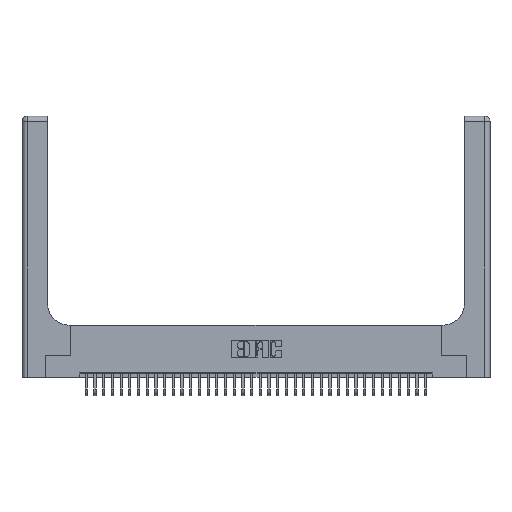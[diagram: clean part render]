
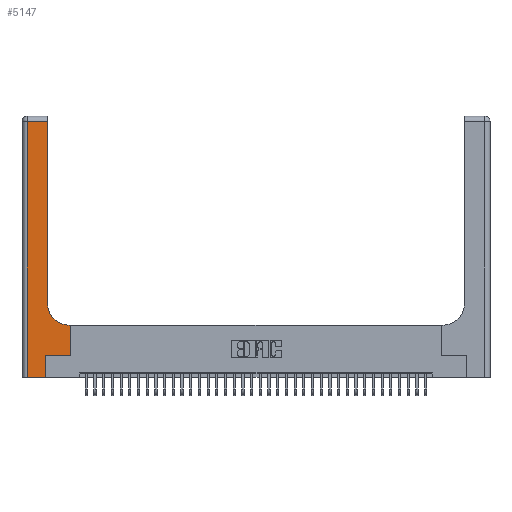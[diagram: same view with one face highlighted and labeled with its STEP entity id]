
A CAD part, top view. The second image highlights one B-rep face of the part: STEP entity #5147.
In plain terms, the highlighted planar face has unit normal (0, 0, 1).
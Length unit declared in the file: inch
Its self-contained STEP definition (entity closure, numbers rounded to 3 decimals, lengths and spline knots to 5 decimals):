
#556 = ORIENTED_EDGE ( 'NONE', *, *, #10678, .T. ) ;
#912 = LINE ( 'NONE', #37851, #16051 ) ;
#923 = VERTEX_POINT ( 'NONE', #15321 ) ;
#1822 = DIRECTION ( 'NONE',  ( 0., 0., -1. ) ) ;
#2585 = EDGE_LOOP ( 'NONE', ( #3251, #27436, #12454, #21646, #556, #5728, #13069, #32507, #8912 ) ) ;
#3251 = ORIENTED_EDGE ( 'NONE', *, *, #26439, .T. ) ;
#5147 = ADVANCED_FACE ( 'NONE', ( #26688 ), #20530, .F. ) ;
#5360 = DIRECTION ( 'NONE',  ( 0., -1., 0. ) ) ;
#5602 = CARTESIAN_POINT ( 'NONE',  ( 0., 3., 0.37 ) ) ;
#5684 = VERTEX_POINT ( 'NONE', #32238 ) ;
#5728 = ORIENTED_EDGE ( 'NONE', *, *, #12887, .T. ) ;
#6260 = AXIS2_PLACEMENT_3D ( 'NONE', #5602, #26417, #8618 ) ;
#6368 = CARTESIAN_POINT ( 'NONE',  ( 0.06, 2.94, 0.37 ) ) ;
#6786 = VECTOR ( 'NONE', #36895, 39.37008 ) ;
#8026 = CARTESIAN_POINT ( 'NONE',  ( 0.5585, 0.6, 0.37 ) ) ;
#8618 = DIRECTION ( 'NONE',  ( -1., 0., 0. ) ) ;
#8731 = LINE ( 'NONE', #11930, #15793 ) ;
#8912 = ORIENTED_EDGE ( 'NONE', *, *, #35461, .T. ) ;
#10533 = CARTESIAN_POINT ( 'NONE',  ( 0.5415, 0.6, 0.37 ) ) ;
#10678 = EDGE_CURVE ( 'NONE', #923, #5684, #22399, .T. ) ;
#11016 = VERTEX_POINT ( 'NONE', #31065 ) ;
#11930 = CARTESIAN_POINT ( 'NONE',  ( 0., 0., 0.37 ) ) ;
#12454 = ORIENTED_EDGE ( 'NONE', *, *, #27567, .T. ) ;
#12887 = EDGE_CURVE ( 'NONE', #5684, #34625, #29479, .T. ) ;
#13069 = ORIENTED_EDGE ( 'NONE', *, *, #23343, .T. ) ;
#13852 = DIRECTION ( 'NONE',  ( 0., 1., 0. ) ) ;
#14161 = CARTESIAN_POINT ( 'NONE',  ( 0.2915, 3., 0.37 ) ) ;
#15321 = CARTESIAN_POINT ( 'NONE',  ( 0.269, 0., 0.37 ) ) ;
#15376 = VECTOR ( 'NONE', #13852, 39.37008 ) ;
#15511 = VERTEX_POINT ( 'NONE', #6368 ) ;
#15736 = LINE ( 'NONE', #22284, #6786 ) ;
#15793 = VECTOR ( 'NONE', #35523, 39.37008 ) ;
#15920 = VERTEX_POINT ( 'NONE', #8026 ) ;
#16034 = CARTESIAN_POINT ( 'NONE',  ( 0.5585, 0.25, 0.37 ) ) ;
#16051 = VECTOR ( 'NONE', #5360, 39.37008 ) ;
#17164 = DIRECTION ( 'NONE',  ( 0., 1., 0. ) ) ;
#17400 = VERTEX_POINT ( 'NONE', #10533 ) ;
#18154 = DIRECTION ( 'NONE',  ( -1., 0., 0. ) ) ;
#18803 = CARTESIAN_POINT ( 'NONE',  ( 0.269, 0.25, 0.37 ) ) ;
#19839 = CARTESIAN_POINT ( 'NONE',  ( 0.5415, 0.85, 0.37 ) ) ;
#19888 = CIRCLE ( 'NONE', #32538, 0.25 ) ;
#20530 = PLANE ( 'NONE',  #6260 ) ;
#20801 = VECTOR ( 'NONE', #33389, 39.37008 ) ;
#21004 = CARTESIAN_POINT ( 'NONE',  ( 0.269, 0., 0.37 ) ) ;
#21234 = CARTESIAN_POINT ( 'NONE',  ( 0.06, 0., 0.37 ) ) ;
#21646 = ORIENTED_EDGE ( 'NONE', *, *, #31395, .T. ) ;
#22284 = CARTESIAN_POINT ( 'NONE',  ( 0., 2.94, 0.37 ) ) ;
#22399 = LINE ( 'NONE', #21004, #37078 ) ;
#22784 = DIRECTION ( 'NONE',  ( 1., 0., 0. ) ) ;
#23343 = EDGE_CURVE ( 'NONE', #34625, #15920, #30086, .T. ) ;
#23945 = DIRECTION ( 'NONE',  ( 0., 1., 0. ) ) ;
#25377 = EDGE_CURVE ( 'NONE', #15920, #17400, #35966, .T. ) ;
#25983 = CARTESIAN_POINT ( 'NONE',  ( 0.5585, 0.25, 0.37 ) ) ;
#26417 = DIRECTION ( 'NONE',  ( 0., 0., -1. ) ) ;
#26439 = EDGE_CURVE ( 'NONE', #11016, #37584, #30365, .T. ) ;
#26688 = FACE_OUTER_BOUND ( 'NONE', #2585, .T. ) ;
#27436 = ORIENTED_EDGE ( 'NONE', *, *, #35345, .T. ) ;
#27567 = EDGE_CURVE ( 'NONE', #15511, #32741, #912, .T. ) ;
#29450 = VECTOR ( 'NONE', #17164, 39.37008 ) ;
#29479 = LINE ( 'NONE', #18803, #20801 ) ;
#29808 = CARTESIAN_POINT ( 'NONE',  ( 0.2915, 0.6, 0.37 ) ) ;
#30086 = LINE ( 'NONE', #25983, #15376 ) ;
#30365 = LINE ( 'NONE', #14161, #29450 ) ;
#31065 = CARTESIAN_POINT ( 'NONE',  ( 0.2915, 0.85, 0.37 ) ) ;
#31395 = EDGE_CURVE ( 'NONE', #32741, #923, #8731, .T. ) ;
#32238 = CARTESIAN_POINT ( 'NONE',  ( 0.269, 0.25, 0.37 ) ) ;
#32507 = ORIENTED_EDGE ( 'NONE', *, *, #25377, .T. ) ;
#32538 = AXIS2_PLACEMENT_3D ( 'NONE', #19839, #1822, #22784 ) ;
#32741 = VERTEX_POINT ( 'NONE', #21234 ) ;
#33389 = DIRECTION ( 'NONE',  ( 1., 0., 0. ) ) ;
#34625 = VERTEX_POINT ( 'NONE', #16034 ) ;
#35036 = VECTOR ( 'NONE', #18154, 39.37008 ) ;
#35345 = EDGE_CURVE ( 'NONE', #37584, #15511, #15736, .T. ) ;
#35461 = EDGE_CURVE ( 'NONE', #17400, #11016, #19888, .T. ) ;
#35523 = DIRECTION ( 'NONE',  ( 1., 0., 0. ) ) ;
#35966 = LINE ( 'NONE', #29808, #35036 ) ;
#36895 = DIRECTION ( 'NONE',  ( -1., 0., 0. ) ) ;
#37078 = VECTOR ( 'NONE', #23945, 39.37008 ) ;
#37483 = CARTESIAN_POINT ( 'NONE',  ( 0.2915, 2.94, 0.37 ) ) ;
#37584 = VERTEX_POINT ( 'NONE', #37483 ) ;
#37851 = CARTESIAN_POINT ( 'NONE',  ( 0.06, 3., 0.37 ) ) ;
